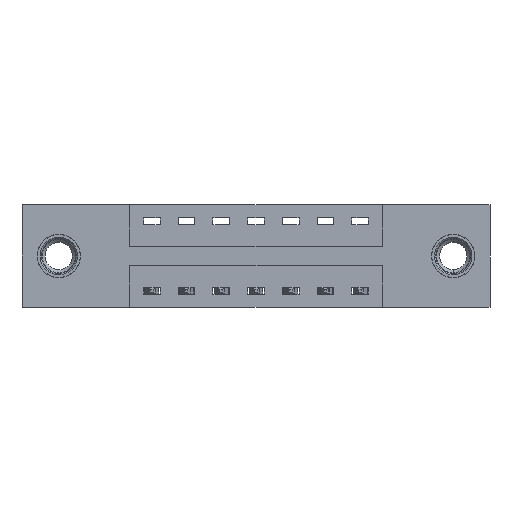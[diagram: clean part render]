
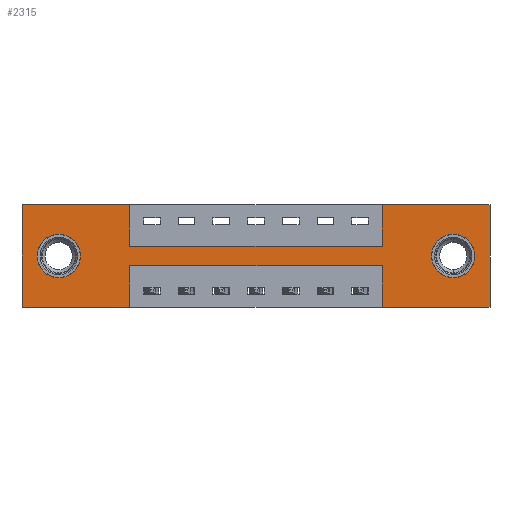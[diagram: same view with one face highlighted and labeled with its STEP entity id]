
A CAD part, front view. The second image highlights one B-rep face of the part: STEP entity #2315.
In plain terms, the highlighted planar face has unit normal (0, -1, 0).
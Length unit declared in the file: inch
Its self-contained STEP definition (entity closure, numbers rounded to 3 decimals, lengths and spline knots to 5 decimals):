
#18 = ORIENTED_EDGE ( 'NONE', *, *, #5357, .F. ) ;
#50 = AXIS2_PLACEMENT_3D ( 'NONE', #6711, #1986, #7507 ) ;
#54 = VERTEX_POINT ( 'NONE', #6367 ) ;
#130 = DIRECTION ( 'NONE',  ( 0., 0., -1. ) ) ;
#148 = LINE ( 'NONE', #331, #9945 ) ;
#168 = CARTESIAN_POINT ( 'NONE',  ( 1.5525, 0., -0.107 ) ) ;
#189 = ORIENTED_EDGE ( 'NONE', *, *, #5695, .F. ) ;
#199 = VECTOR ( 'NONE', #6383, 39.37008 ) ;
#216 = VERTEX_POINT ( 'NONE', #168 ) ;
#331 = CARTESIAN_POINT ( 'NONE',  ( 0., 0., 0. ) ) ;
#509 = CARTESIAN_POINT ( 'NONE',  ( 0.3875, 0., -0.22 ) ) ;
#695 = DIRECTION ( 'NONE',  ( -1., 0., 0. ) ) ;
#854 = VERTEX_POINT ( 'NONE', #5728 ) ;
#921 = CARTESIAN_POINT ( 'NONE',  ( 0.3875, 0., 0. ) ) ;
#982 = CIRCLE ( 'NONE', #50, 0.078 ) ;
#1087 = VECTOR ( 'NONE', #7417, 39.37008 ) ;
#1207 = FACE_OUTER_BOUND ( 'NONE', #4020, .T. ) ;
#1243 = DIRECTION ( 'NONE',  ( 0., 1., 0. ) ) ;
#1354 = CARTESIAN_POINT ( 'NONE',  ( 0.3875, 0., -0.37 ) ) ;
#1552 = DIRECTION ( 'NONE',  ( 0., 0., 1. ) ) ;
#1553 = EDGE_LOOP ( 'NONE', ( #5388, #2440 ) ) ;
#1674 = EDGE_LOOP ( 'NONE', ( #1831, #1948 ) ) ;
#1712 = DIRECTION ( 'NONE',  ( 0., 0., 1. ) ) ;
#1726 = LINE ( 'NONE', #7986, #3576 ) ;
#1733 = CIRCLE ( 'NONE', #7680, 0.078 ) ;
#1773 = CARTESIAN_POINT ( 'NONE',  ( 1.5525, 0., -0.263 ) ) ;
#1831 = ORIENTED_EDGE ( 'NONE', *, *, #7576, .T. ) ;
#1836 = VECTOR ( 'NONE', #3390, 39.37008 ) ;
#1938 = DIRECTION ( 'NONE',  ( 1., 0., 0. ) ) ;
#1948 = ORIENTED_EDGE ( 'NONE', *, *, #7679, .T. ) ;
#1981 = VERTEX_POINT ( 'NONE', #1773 ) ;
#1986 = DIRECTION ( 'NONE',  ( 0., 1., 0. ) ) ;
#1997 = EDGE_CURVE ( 'NONE', #9347, #3665, #9998, .T. ) ;
#2018 = CARTESIAN_POINT ( 'NONE',  ( 0.1325, 0., -0.107 ) ) ;
#2075 = EDGE_CURVE ( 'NONE', #54, #9900, #9503, .T. ) ;
#2315 = ADVANCED_FACE ( 'NONE', ( #9369, #9872, #1207 ), #7068, .T. ) ;
#2337 = EDGE_CURVE ( 'NONE', #3047, #4127, #9118, .T. ) ;
#2410 = EDGE_CURVE ( 'NONE', #854, #7421, #6505, .T. ) ;
#2422 = VERTEX_POINT ( 'NONE', #4822 ) ;
#2440 = ORIENTED_EDGE ( 'NONE', *, *, #8134, .T. ) ;
#2521 = DIRECTION ( 'NONE',  ( 0., 1., 0. ) ) ;
#2552 = CARTESIAN_POINT ( 'NONE',  ( 0.3875, 0., -0.15 ) ) ;
#2656 = EDGE_CURVE ( 'NONE', #216, #1981, #6627, .T. ) ;
#2821 = VECTOR ( 'NONE', #7867, 39.37008 ) ;
#2955 = LINE ( 'NONE', #509, #5035 ) ;
#3003 = LINE ( 'NONE', #6152, #9048 ) ;
#3047 = VERTEX_POINT ( 'NONE', #3302 ) ;
#3206 = VERTEX_POINT ( 'NONE', #9032 ) ;
#3281 = ORIENTED_EDGE ( 'NONE', *, *, #8862, .F. ) ;
#3302 = CARTESIAN_POINT ( 'NONE',  ( 1.685, 0., -0.37 ) ) ;
#3374 = VECTOR ( 'NONE', #8773, 39.37008 ) ;
#3390 = DIRECTION ( 'NONE',  ( 1., 0., 0. ) ) ;
#3501 = ORIENTED_EDGE ( 'NONE', *, *, #1997, .F. ) ;
#3558 = DIRECTION ( 'NONE',  ( 0., 0., -1. ) ) ;
#3574 = DIRECTION ( 'NONE',  ( 0., 0., 1. ) ) ;
#3576 = VECTOR ( 'NONE', #1712, 39.37008 ) ;
#3665 = VERTEX_POINT ( 'NONE', #4831 ) ;
#3773 = DIRECTION ( 'NONE',  ( 0., 0., -1. ) ) ;
#3895 = CARTESIAN_POINT ( 'NONE',  ( 1.2975, 0., 0. ) ) ;
#3935 = DIRECTION ( 'NONE',  ( 0., -1., 0. ) ) ;
#4020 = EDGE_LOOP ( 'NONE', ( #4691, #3281, #8434, #4068, #7023, #6029, #189, #3501, #18, #7325, #9683, #5867 ) ) ;
#4030 = VERTEX_POINT ( 'NONE', #1354 ) ;
#4068 = ORIENTED_EDGE ( 'NONE', *, *, #2337, .F. ) ;
#4110 = AXIS2_PLACEMENT_3D ( 'NONE', #9617, #4865, #130 ) ;
#4127 = VERTEX_POINT ( 'NONE', #9364 ) ;
#4329 = VERTEX_POINT ( 'NONE', #921 ) ;
#4604 = LINE ( 'NONE', #3895, #4843 ) ;
#4691 = ORIENTED_EDGE ( 'NONE', *, *, #5836, .F. ) ;
#4732 = CARTESIAN_POINT ( 'NONE',  ( 1.685, 0., 0. ) ) ;
#4776 = VERTEX_POINT ( 'NONE', #2018 ) ;
#4822 = CARTESIAN_POINT ( 'NONE',  ( 0.3875, 0., -0.22 ) ) ;
#4831 = CARTESIAN_POINT ( 'NONE',  ( 1.2975, 0., -0.15 ) ) ;
#4843 = VECTOR ( 'NONE', #1552, 39.37008 ) ;
#4865 = DIRECTION ( 'NONE',  ( 0., 1., 0. ) ) ;
#5035 = VECTOR ( 'NONE', #6839, 39.37008 ) ;
#5319 = EDGE_CURVE ( 'NONE', #7421, #4329, #148, .T. ) ;
#5357 = EDGE_CURVE ( 'NONE', #4329, #9347, #7575, .T. ) ;
#5388 = ORIENTED_EDGE ( 'NONE', *, *, #2656, .T. ) ;
#5695 = EDGE_CURVE ( 'NONE', #3665, #54, #4604, .T. ) ;
#5728 = CARTESIAN_POINT ( 'NONE',  ( 0., 0., -0.37 ) ) ;
#5749 = CARTESIAN_POINT ( 'NONE',  ( 1.2975, 0., -0.22 ) ) ;
#5836 = EDGE_CURVE ( 'NONE', #2422, #4030, #9684, .T. ) ;
#5867 = ORIENTED_EDGE ( 'NONE', *, *, #7945, .F. ) ;
#5919 = VERTEX_POINT ( 'NONE', #5749 ) ;
#5967 = CARTESIAN_POINT ( 'NONE',  ( 1.5525, 0., -0.185 ) ) ;
#6029 = ORIENTED_EDGE ( 'NONE', *, *, #2075, .F. ) ;
#6152 = CARTESIAN_POINT ( 'NONE',  ( 1.685, 0., 0. ) ) ;
#6367 = CARTESIAN_POINT ( 'NONE',  ( 1.2975, 0., 0. ) ) ;
#6383 = DIRECTION ( 'NONE',  ( 0., 0., 1. ) ) ;
#6407 = VECTOR ( 'NONE', #695, 39.37008 ) ;
#6505 = LINE ( 'NONE', #7170, #199 ) ;
#6627 = CIRCLE ( 'NONE', #7173, 0.078 ) ;
#6711 = CARTESIAN_POINT ( 'NONE',  ( 0.1325, 0., -0.185 ) ) ;
#6758 = DIRECTION ( 'NONE',  ( 0., 0., -1. ) ) ;
#6839 = DIRECTION ( 'NONE',  ( -1., 0., 0. ) ) ;
#7019 = CIRCLE ( 'NONE', #4110, 0.078 ) ;
#7023 = ORIENTED_EDGE ( 'NONE', *, *, #8501, .F. ) ;
#7068 = PLANE ( 'NONE',  #9513 ) ;
#7103 = CARTESIAN_POINT ( 'NONE',  ( 0., 0., -0.37 ) ) ;
#7170 = CARTESIAN_POINT ( 'NONE',  ( 0., 0., 0. ) ) ;
#7173 = AXIS2_PLACEMENT_3D ( 'NONE', #5967, #1243, #6758 ) ;
#7231 = CARTESIAN_POINT ( 'NONE',  ( 0.1325, 0., -0.185 ) ) ;
#7325 = ORIENTED_EDGE ( 'NONE', *, *, #5319, .F. ) ;
#7417 = DIRECTION ( 'NONE',  ( 1., 0., 0. ) ) ;
#7421 = VERTEX_POINT ( 'NONE', #9359 ) ;
#7507 = DIRECTION ( 'NONE',  ( 0., 0., 1. ) ) ;
#7575 = LINE ( 'NONE', #8303, #7828 ) ;
#7576 = EDGE_CURVE ( 'NONE', #4776, #3206, #1733, .T. ) ;
#7679 = EDGE_CURVE ( 'NONE', #3206, #4776, #982, .T. ) ;
#7680 = AXIS2_PLACEMENT_3D ( 'NONE', #7231, #2521, #3574 ) ;
#7828 = VECTOR ( 'NONE', #3558, 39.37008 ) ;
#7867 = DIRECTION ( 'NONE',  ( -1., 0., 0. ) ) ;
#7945 = EDGE_CURVE ( 'NONE', #4030, #854, #8772, .T. ) ;
#7986 = CARTESIAN_POINT ( 'NONE',  ( 1.2975, 0., -0.37 ) ) ;
#7998 = CARTESIAN_POINT ( 'NONE',  ( 0.3875, 0., -0.37 ) ) ;
#8122 = CARTESIAN_POINT ( 'NONE',  ( 0.3875, 0., -0.15 ) ) ;
#8134 = EDGE_CURVE ( 'NONE', #1981, #216, #7019, .T. ) ;
#8303 = CARTESIAN_POINT ( 'NONE',  ( 0.3875, 0., 0. ) ) ;
#8434 = ORIENTED_EDGE ( 'NONE', *, *, #9952, .F. ) ;
#8501 = EDGE_CURVE ( 'NONE', #9900, #3047, #3003, .T. ) ;
#8587 = CARTESIAN_POINT ( 'NONE',  ( 0., 0., -0.37 ) ) ;
#8675 = CARTESIAN_POINT ( 'NONE',  ( 0., 0., -0.37 ) ) ;
#8772 = LINE ( 'NONE', #8587, #6407 ) ;
#8773 = DIRECTION ( 'NONE',  ( 0., 0., -1. ) ) ;
#8862 = EDGE_CURVE ( 'NONE', #5919, #2422, #2955, .T. ) ;
#9016 = CARTESIAN_POINT ( 'NONE',  ( 0., 0., 0. ) ) ;
#9032 = CARTESIAN_POINT ( 'NONE',  ( 0.1325, 0., -0.263 ) ) ;
#9048 = VECTOR ( 'NONE', #3773, 39.37008 ) ;
#9118 = LINE ( 'NONE', #7103, #2821 ) ;
#9347 = VERTEX_POINT ( 'NONE', #2552 ) ;
#9359 = CARTESIAN_POINT ( 'NONE',  ( 0., 0., 0. ) ) ;
#9364 = CARTESIAN_POINT ( 'NONE',  ( 1.2975, 0., -0.37 ) ) ;
#9369 = FACE_BOUND ( 'NONE', #1553, .T. ) ;
#9475 = DIRECTION ( 'NONE',  ( 0., 0., -1. ) ) ;
#9503 = LINE ( 'NONE', #9016, #1087 ) ;
#9513 = AXIS2_PLACEMENT_3D ( 'NONE', #8675, #3935, #9475 ) ;
#9617 = CARTESIAN_POINT ( 'NONE',  ( 1.5525, 0., -0.185 ) ) ;
#9683 = ORIENTED_EDGE ( 'NONE', *, *, #2410, .F. ) ;
#9684 = LINE ( 'NONE', #7998, #3374 ) ;
#9872 = FACE_BOUND ( 'NONE', #1674, .T. ) ;
#9900 = VERTEX_POINT ( 'NONE', #4732 ) ;
#9945 = VECTOR ( 'NONE', #1938, 39.37008 ) ;
#9952 = EDGE_CURVE ( 'NONE', #4127, #5919, #1726, .T. ) ;
#9998 = LINE ( 'NONE', #8122, #1836 ) ;
